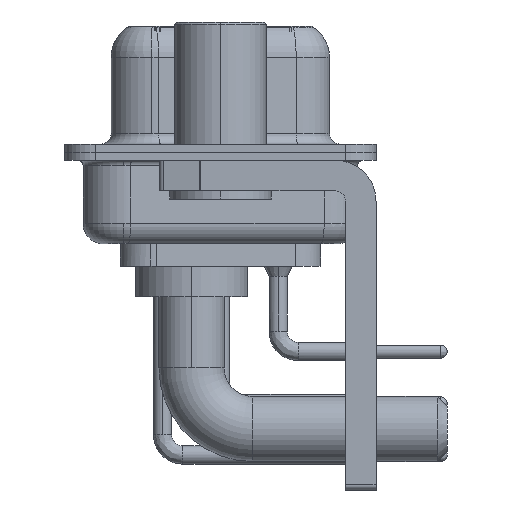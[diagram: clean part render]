
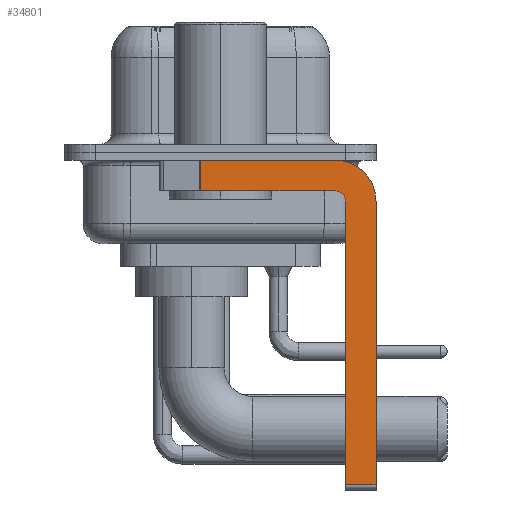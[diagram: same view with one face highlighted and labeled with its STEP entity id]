
A CAD part, left-side view. The second image highlights one B-rep face of the part: STEP entity #34801.
In plain terms, the highlighted planar face has unit normal (-1, 0, 0).
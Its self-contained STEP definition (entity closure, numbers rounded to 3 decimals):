
#111 = PLANE ( 'NONE',  #30669 ) ;
#1747 = CARTESIAN_POINT ( 'NONE',  ( -2.9, -7.65, -16.35 ) ) ;
#2074 = CIRCLE ( 'NONE', #21229, 0.5 ) ;
#2854 = ORIENTED_EDGE ( 'NONE', *, *, #34632, .F. ) ;
#3415 = ORIENTED_EDGE ( 'NONE', *, *, #21352, .F. ) ;
#3894 = DIRECTION ( 'NONE',  ( 0., 1., 0. ) ) ;
#5747 = DIRECTION ( 'NONE',  ( 0., 0., -1. ) ) ;
#5988 = EDGE_CURVE ( 'NONE', #34863, #18796, #20016, .T. ) ;
#6306 = VECTOR ( 'NONE', #3894, 1000. ) ;
#7230 = ORIENTED_EDGE ( 'NONE', *, *, #23399, .F. ) ;
#8269 = FACE_OUTER_BOUND ( 'NONE', #16986, .T. ) ;
#9346 = VERTEX_POINT ( 'NONE', #26831 ) ;
#9919 = CARTESIAN_POINT ( 'NONE',  ( -2.9, -5.65, -16.35 ) ) ;
#10060 = CARTESIAN_POINT ( 'NONE',  ( -2.9, -6.15, -16.35 ) ) ;
#10279 = DIRECTION ( 'NONE',  ( -1., 0., 0. ) ) ;
#11053 = CARTESIAN_POINT ( 'NONE',  ( -2.9, 0.978, -1.9 ) ) ;
#11339 = CARTESIAN_POINT ( 'NONE',  ( -2.9, 3., -0.4 ) ) ;
#12092 = VECTOR ( 'NONE', #20742, 1000. ) ;
#12596 = LINE ( 'NONE', #15588, #14566 ) ;
#13041 = EDGE_CURVE ( 'NONE', #20702, #30625, #13842, .T. ) ;
#13132 = DIRECTION ( 'NONE',  ( 0., 0., 1. ) ) ;
#13270 = VERTEX_POINT ( 'NONE', #11053 ) ;
#13361 = VECTOR ( 'NONE', #24994, 1000. ) ;
#13842 = LINE ( 'NONE', #26782, #22785 ) ;
#13931 = DIRECTION ( 'NONE',  ( 1., 0., 0. ) ) ;
#14019 = EDGE_CURVE ( 'NONE', #20702, #22875, #24094, .T. ) ;
#14124 = ORIENTED_EDGE ( 'NONE', *, *, #5988, .F. ) ;
#14566 = VECTOR ( 'NONE', #18772, 1000. ) ;
#15588 = CARTESIAN_POINT ( 'NONE',  ( -2.9, 0.978, -1.9 ) ) ;
#16050 = CARTESIAN_POINT ( 'NONE',  ( -2.9, 0.978, -0.4 ) ) ;
#16082 = AXIS2_PLACEMENT_3D ( 'NONE', #25472, #17316, #20668 ) ;
#16229 = DIRECTION ( 'NONE',  ( 0., 0., -1. ) ) ;
#16511 = CARTESIAN_POINT ( 'NONE',  ( -2.9, -7.65, -2.4 ) ) ;
#16650 = ORIENTED_EDGE ( 'NONE', *, *, #13041, .F. ) ;
#16733 = EDGE_CURVE ( 'NONE', #30625, #9346, #2074, .T. ) ;
#16986 = EDGE_LOOP ( 'NONE', ( #14124, #19156, #2854, #21553, #16650, #18400, #3415, #7230 ) ) ;
#17245 = CIRCLE ( 'NONE', #16082, 2. ) ;
#17316 = DIRECTION ( 'NONE',  ( 1., 0., 0. ) ) ;
#17328 = CARTESIAN_POINT ( 'NONE',  ( -2.9, -5.65, -1.9 ) ) ;
#18400 = ORIENTED_EDGE ( 'NONE', *, *, #14019, .T. ) ;
#18606 = DIRECTION ( 'NONE',  ( 0., 0., 1. ) ) ;
#18772 = DIRECTION ( 'NONE',  ( 0., 0., -1. ) ) ;
#18796 = VERTEX_POINT ( 'NONE', #30891 ) ;
#18999 = EDGE_CURVE ( 'NONE', #34863, #13270, #12596, .T. ) ;
#19156 = ORIENTED_EDGE ( 'NONE', *, *, #18999, .T. ) ;
#19891 = CARTESIAN_POINT ( 'NONE',  ( -2.9, -7.65, -2.4 ) ) ;
#20016 = LINE ( 'NONE', #11339, #13361 ) ;
#20518 = VECTOR ( 'NONE', #5747, 1000. ) ;
#20668 = DIRECTION ( 'NONE',  ( 0., 0., -1. ) ) ;
#20702 = VERTEX_POINT ( 'NONE', #10060 ) ;
#20742 = DIRECTION ( 'NONE',  ( 0., -1., 0. ) ) ;
#21229 = AXIS2_PLACEMENT_3D ( 'NONE', #34759, #10279, #18606 ) ;
#21352 = EDGE_CURVE ( 'NONE', #23897, #22875, #30013, .T. ) ;
#21368 = CARTESIAN_POINT ( 'NONE',  ( -2.9, -5.65, -2.4 ) ) ;
#21553 = ORIENTED_EDGE ( 'NONE', *, *, #16733, .F. ) ;
#22785 = VECTOR ( 'NONE', #13132, 1000. ) ;
#22875 = VERTEX_POINT ( 'NONE', #1747 ) ;
#23399 = EDGE_CURVE ( 'NONE', #18796, #23897, #17245, .T. ) ;
#23897 = VERTEX_POINT ( 'NONE', #16511 ) ;
#24094 = LINE ( 'NONE', #9919, #12092 ) ;
#24994 = DIRECTION ( 'NONE',  ( 0., -1., 0. ) ) ;
#25061 = CARTESIAN_POINT ( 'NONE',  ( -2.9, -6.15, -2.4 ) ) ;
#25472 = CARTESIAN_POINT ( 'NONE',  ( -2.9, -5.65, -2.4 ) ) ;
#26782 = CARTESIAN_POINT ( 'NONE',  ( -2.9, -6.15, -16.6 ) ) ;
#26831 = CARTESIAN_POINT ( 'NONE',  ( -2.9, -5.65, -1.9 ) ) ;
#30013 = LINE ( 'NONE', #19891, #20518 ) ;
#30625 = VERTEX_POINT ( 'NONE', #25061 ) ;
#30669 = AXIS2_PLACEMENT_3D ( 'NONE', #21368, #13931, #16229 ) ;
#30891 = CARTESIAN_POINT ( 'NONE',  ( -2.9, -5.65, -0.4 ) ) ;
#33137 = LINE ( 'NONE', #17328, #6306 ) ;
#34632 = EDGE_CURVE ( 'NONE', #9346, #13270, #33137, .T. ) ;
#34759 = CARTESIAN_POINT ( 'NONE',  ( -2.9, -5.65, -2.4 ) ) ;
#34801 = ADVANCED_FACE ( 'NONE', ( #8269 ), #111, .F. ) ;
#34863 = VERTEX_POINT ( 'NONE', #16050 ) ;
